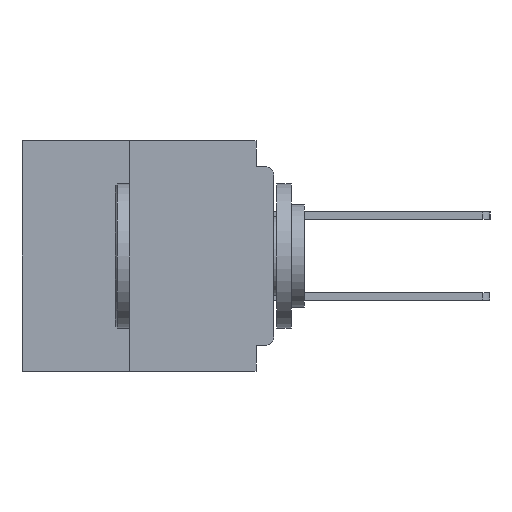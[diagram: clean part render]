
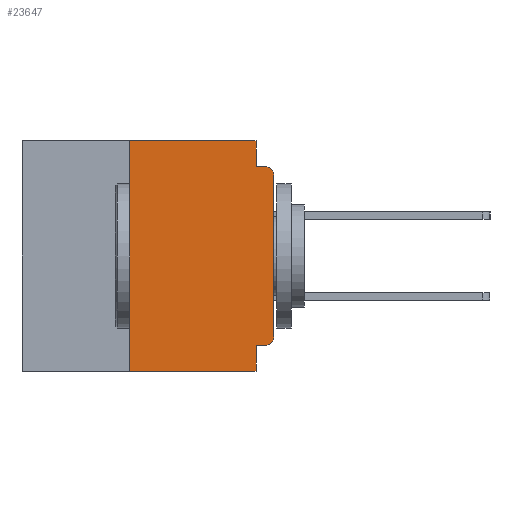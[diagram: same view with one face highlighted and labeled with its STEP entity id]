
A CAD part, left-side view. The second image highlights one B-rep face of the part: STEP entity #23647.
In plain terms, the highlighted planar face has unit normal (-1, 0, 0).
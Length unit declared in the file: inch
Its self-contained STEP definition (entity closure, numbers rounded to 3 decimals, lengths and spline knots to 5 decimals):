
#397 = EDGE_CURVE ( 'NONE', #9535, #44952, #26226, .T. ) ;
#1478 = DIRECTION ( 'NONE',  ( 0., -1., 0. ) ) ;
#2212 = EDGE_CURVE ( 'NONE', #9535, #4640, #29178, .T. ) ;
#2353 = DIRECTION ( 'NONE',  ( 0., 0., -1. ) ) ;
#2508 = CARTESIAN_POINT ( 'NONE',  ( 0., 0.437, -0.4 ) ) ;
#2509 = DIRECTION ( 'NONE',  ( -1., 0., 0. ) ) ;
#2520 = CARTESIAN_POINT ( 'NONE',  ( 0., 0.015, -0.34 ) ) ;
#3962 = CARTESIAN_POINT ( 'NONE',  ( 0., 0., -0.34 ) ) ;
#4640 = VERTEX_POINT ( 'NONE', #3962 ) ;
#4803 = CIRCLE ( 'NONE', #21660, 0.015 ) ;
#6173 = CARTESIAN_POINT ( 'NONE',  ( 0., 0., 0. ) ) ;
#7489 = PLANE ( 'NONE',  #12729 ) ;
#7638 = DIRECTION ( 'NONE',  ( 1., 0., 0. ) ) ;
#7837 = CARTESIAN_POINT ( 'NONE',  ( 0., 0.015, -0.355 ) ) ;
#8979 = VECTOR ( 'NONE', #29652, 39.37008 ) ;
#9535 = VERTEX_POINT ( 'NONE', #7837 ) ;
#10172 = LINE ( 'NONE', #2508, #26751 ) ;
#10723 = VERTEX_POINT ( 'NONE', #18987 ) ;
#10786 = EDGE_CURVE ( 'NONE', #27761, #10723, #29700, .T. ) ;
#11267 = EDGE_LOOP ( 'NONE', ( #36388, #29108, #33007, #19991, #43604, #15303, #19329, #21449, #44190, #17726 ) ) ;
#12151 = VERTEX_POINT ( 'NONE', #29907 ) ;
#12729 = AXIS2_PLACEMENT_3D ( 'NONE', #21779, #7638, #32341 ) ;
#14171 = VECTOR ( 'NONE', #27345, 39.37008 ) ;
#14414 = DIRECTION ( 'NONE',  ( 0., 0., -1. ) ) ;
#14816 = VECTOR ( 'NONE', #1478, 39.37008 ) ;
#15303 = ORIENTED_EDGE ( 'NONE', *, *, #24219, .F. ) ;
#16444 = VERTEX_POINT ( 'NONE', #44995 ) ;
#16632 = DIRECTION ( 'NONE',  ( 0., -1., 0. ) ) ;
#17726 = ORIENTED_EDGE ( 'NONE', *, *, #2212, .T. ) ;
#17950 = VECTOR ( 'NONE', #35500, 39.37008 ) ;
#18469 = LINE ( 'NONE', #36385, #8979 ) ;
#18578 = VERTEX_POINT ( 'NONE', #22487 ) ;
#18987 = CARTESIAN_POINT ( 'NONE',  ( 0., 0.031, -0.045 ) ) ;
#19311 = CARTESIAN_POINT ( 'NONE',  ( 0., 0.015, -0.06 ) ) ;
#19329 = ORIENTED_EDGE ( 'NONE', *, *, #24003, .T. ) ;
#19991 = ORIENTED_EDGE ( 'NONE', *, *, #10786, .F. ) ;
#21402 = LINE ( 'NONE', #6173, #14171 ) ;
#21449 = ORIENTED_EDGE ( 'NONE', *, *, #26742, .F. ) ;
#21509 = VECTOR ( 'NONE', #40180, 39.37008 ) ;
#21660 = AXIS2_PLACEMENT_3D ( 'NONE', #19311, #43628, #22844 ) ;
#21779 = CARTESIAN_POINT ( 'NONE',  ( 0., 0.437, 0. ) ) ;
#22487 = CARTESIAN_POINT ( 'NONE',  ( 0., 0.25, -0.4 ) ) ;
#22532 = CARTESIAN_POINT ( 'NONE',  ( 0., 0., -0.06 ) ) ;
#22823 = CARTESIAN_POINT ( 'NONE',  ( 0., 0.031, 0. ) ) ;
#22844 = DIRECTION ( 'NONE',  ( 0., 0., -1. ) ) ;
#22848 = EDGE_CURVE ( 'NONE', #4640, #23766, #21402, .T. ) ;
#23481 = VERTEX_POINT ( 'NONE', #27927 ) ;
#23497 = FACE_OUTER_BOUND ( 'NONE', #11267, .T. ) ;
#23647 = ADVANCED_FACE ( 'NONE', ( #23497 ), #7489, .F. ) ;
#23766 = VERTEX_POINT ( 'NONE', #22532 ) ;
#24003 = EDGE_CURVE ( 'NONE', #18578, #12151, #10172, .T. ) ;
#24219 = EDGE_CURVE ( 'NONE', #18578, #16444, #36560, .T. ) ;
#24250 = LINE ( 'NONE', #29568, #14816 ) ;
#24415 = EDGE_CURVE ( 'NONE', #16444, #27761, #18469, .T. ) ;
#26226 = LINE ( 'NONE', #28881, #43554 ) ;
#26742 = EDGE_CURVE ( 'NONE', #44952, #12151, #42617, .T. ) ;
#26751 = VECTOR ( 'NONE', #16632, 39.37008 ) ;
#27345 = DIRECTION ( 'NONE',  ( 0., 0., 1. ) ) ;
#27704 = CARTESIAN_POINT ( 'NONE',  ( 0., 0.031, 0. ) ) ;
#27761 = VERTEX_POINT ( 'NONE', #27704 ) ;
#27927 = CARTESIAN_POINT ( 'NONE',  ( 0., 0.015, -0.045 ) ) ;
#28881 = CARTESIAN_POINT ( 'NONE',  ( 0., 0., -0.355 ) ) ;
#29108 = ORIENTED_EDGE ( 'NONE', *, *, #40319, .T. ) ;
#29178 = CIRCLE ( 'NONE', #30083, 0.015 ) ;
#29568 = CARTESIAN_POINT ( 'NONE',  ( 0., 0., -0.045 ) ) ;
#29652 = DIRECTION ( 'NONE',  ( 0., -1., 0. ) ) ;
#29700 = LINE ( 'NONE', #22823, #21509 ) ;
#29907 = CARTESIAN_POINT ( 'NONE',  ( 0., 0.031, -0.4 ) ) ;
#30083 = AXIS2_PLACEMENT_3D ( 'NONE', #2520, #2509, #2353 ) ;
#31938 = EDGE_CURVE ( 'NONE', #10723, #23481, #24250, .T. ) ;
#31986 = CARTESIAN_POINT ( 'NONE',  ( 0., 0.25, -0.4 ) ) ;
#32341 = DIRECTION ( 'NONE',  ( 0., 0., -1. ) ) ;
#32507 = DIRECTION ( 'NONE',  ( 0., 1., 0. ) ) ;
#33007 = ORIENTED_EDGE ( 'NONE', *, *, #31938, .F. ) ;
#34481 = CARTESIAN_POINT ( 'NONE',  ( 0., 0.031, -0.355 ) ) ;
#35487 = CARTESIAN_POINT ( 'NONE',  ( 0., 0.031, -0.4 ) ) ;
#35500 = DIRECTION ( 'NONE',  ( 0., 0., 1. ) ) ;
#36385 = CARTESIAN_POINT ( 'NONE',  ( 0., 0.437, 0. ) ) ;
#36388 = ORIENTED_EDGE ( 'NONE', *, *, #22848, .T. ) ;
#36560 = LINE ( 'NONE', #31986, #17950 ) ;
#40180 = DIRECTION ( 'NONE',  ( 0., 0., -1. ) ) ;
#40319 = EDGE_CURVE ( 'NONE', #23766, #23481, #4803, .T. ) ;
#42617 = LINE ( 'NONE', #35487, #43667 ) ;
#43554 = VECTOR ( 'NONE', #32507, 39.37008 ) ;
#43604 = ORIENTED_EDGE ( 'NONE', *, *, #24415, .F. ) ;
#43628 = DIRECTION ( 'NONE',  ( -1., 0., 0. ) ) ;
#43667 = VECTOR ( 'NONE', #14414, 39.37008 ) ;
#44190 = ORIENTED_EDGE ( 'NONE', *, *, #397, .F. ) ;
#44952 = VERTEX_POINT ( 'NONE', #34481 ) ;
#44995 = CARTESIAN_POINT ( 'NONE',  ( 0., 0.25, 0. ) ) ;
